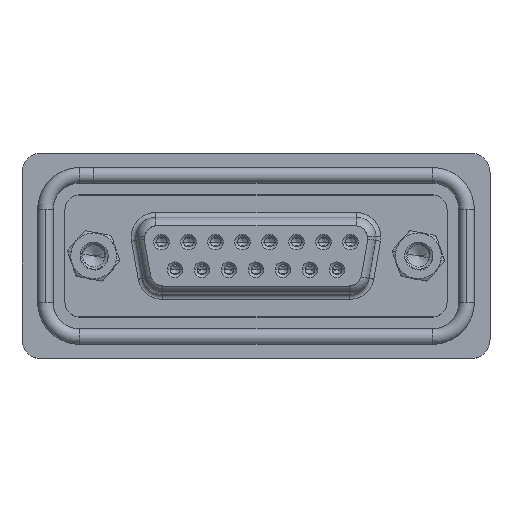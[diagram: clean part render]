
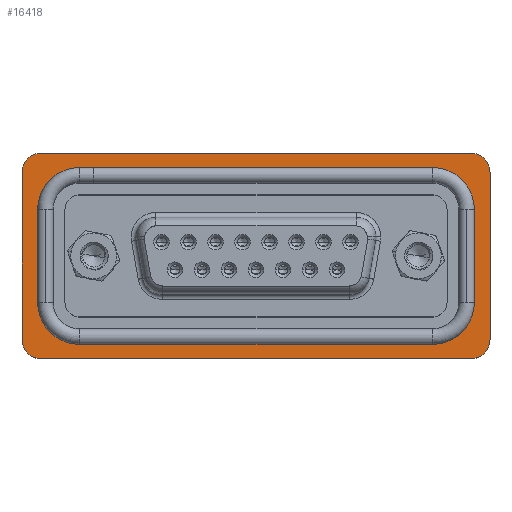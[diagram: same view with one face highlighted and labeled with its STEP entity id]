
A CAD part, top view. The second image highlights one B-rep face of the part: STEP entity #16418.
In plain terms, the highlighted planar face has unit normal (0, 0, 1).
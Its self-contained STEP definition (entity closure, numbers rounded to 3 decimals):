
#481 = VERTEX_POINT ( 'NONE', #18324 ) ;
#575 = DIRECTION ( 'NONE',  ( 1., 0., 0. ) ) ;
#1080 = CARTESIAN_POINT ( 'NONE',  ( 34.75, 9.075, 0.5 ) ) ;
#1160 = VERTEX_POINT ( 'NONE', #1566 ) ;
#1203 = CARTESIAN_POINT ( 'NONE',  ( -1.45, -9.075, 0.5 ) ) ;
#1566 = CARTESIAN_POINT ( 'NONE',  ( -5.75, 4.775, 0.5 ) ) ;
#1603 = ORIENTED_EDGE ( 'NONE', *, *, #8219, .T. ) ;
#1607 = ORIENTED_EDGE ( 'NONE', *, *, #5086, .F. ) ;
#1624 = CARTESIAN_POINT ( 'NONE',  ( -5.75, 4.775, 0.5 ) ) ;
#2034 = EDGE_CURVE ( 'NONE', #1160, #13323, #21822, .T. ) ;
#2039 = EDGE_CURVE ( 'NONE', #20120, #16101, #14316, .T. ) ;
#2099 = DIRECTION ( 'NONE',  ( 1., 0., 0. ) ) ;
#2101 = DIRECTION ( 'NONE',  ( 0., 1., 0. ) ) ;
#2139 = CIRCLE ( 'NONE', #2928, 2. ) ;
#2326 = CIRCLE ( 'NONE', #15677, 4.3 ) ;
#2415 = PLANE ( 'NONE',  #2941 ) ;
#2778 = VERTEX_POINT ( 'NONE', #7340 ) ;
#2786 = VERTEX_POINT ( 'NONE', #23828 ) ;
#2828 = DIRECTION ( 'NONE',  ( 1., 0., 0. ) ) ;
#2928 = AXIS2_PLACEMENT_3D ( 'NONE', #12668, #21630, #3425 ) ;
#2941 = AXIS2_PLACEMENT_3D ( 'NONE', #9953, #17433, #575 ) ;
#3277 = CARTESIAN_POINT ( 'NONE',  ( 40.65, 8.55, 0.5 ) ) ;
#3402 = CARTESIAN_POINT ( 'NONE',  ( 38.65, -10.55, 0.5 ) ) ;
#3425 = DIRECTION ( 'NONE',  ( -1., 0., 0. ) ) ;
#3708 = CARTESIAN_POINT ( 'NONE',  ( 40.65, -8.55, 0.5 ) ) ;
#3929 = VECTOR ( 'NONE', #2101, 1000. ) ;
#4062 = LINE ( 'NONE', #19078, #10665 ) ;
#4229 = CARTESIAN_POINT ( 'NONE',  ( 38.65, -10.55, 0.5 ) ) ;
#4257 = FACE_OUTER_BOUND ( 'NONE', #14804, .T. ) ;
#4296 = DIRECTION ( 'NONE',  ( -1., 0., 0. ) ) ;
#4420 = CARTESIAN_POINT ( 'NONE',  ( 38.65, 8.55, 0.5 ) ) ;
#4846 = DIRECTION ( 'NONE',  ( 0., 0., 1. ) ) ;
#4866 = AXIS2_PLACEMENT_3D ( 'NONE', #10271, #4846, #12354 ) ;
#4886 = ORIENTED_EDGE ( 'NONE', *, *, #23094, .T. ) ;
#5086 = EDGE_CURVE ( 'NONE', #16101, #1160, #18033, .T. ) ;
#5258 = DIRECTION ( 'NONE',  ( 1., 0., 0. ) ) ;
#5280 = AXIS2_PLACEMENT_3D ( 'NONE', #13414, #22400, #18942 ) ;
#5379 = LINE ( 'NONE', #3402, #12160 ) ;
#5762 = CARTESIAN_POINT ( 'NONE',  ( -1.45, 9.075, 0.5 ) ) ;
#5792 = EDGE_CURVE ( 'NONE', #19584, #20791, #5379, .T. ) ;
#6074 = VECTOR ( 'NONE', #11940, 1000. ) ;
#6156 = ORIENTED_EDGE ( 'NONE', *, *, #18414, .T. ) ;
#6298 = VERTEX_POINT ( 'NONE', #10416 ) ;
#6778 = DIRECTION ( 'NONE',  ( 1., 0., 0. ) ) ;
#7009 = DIRECTION ( 'NONE',  ( 1., 0., 0. ) ) ;
#7166 = EDGE_CURVE ( 'NONE', #20648, #23258, #21580, .T. ) ;
#7315 = EDGE_CURVE ( 'NONE', #13323, #2778, #2326, .T. ) ;
#7340 = CARTESIAN_POINT ( 'NONE',  ( -1.45, -9.075, 0.5 ) ) ;
#7544 = LINE ( 'NONE', #3708, #3929 ) ;
#7584 = ORIENTED_EDGE ( 'NONE', *, *, #15736, .F. ) ;
#7915 = DIRECTION ( 'NONE',  ( 0., 0., 1. ) ) ;
#8021 = CARTESIAN_POINT ( 'NONE',  ( -7.35, -8.55, 0.5 ) ) ;
#8147 = CARTESIAN_POINT ( 'NONE',  ( 39.05, -4.775, 0.5 ) ) ;
#8219 = EDGE_CURVE ( 'NONE', #22334, #20648, #7544, .T. ) ;
#8475 = VERTEX_POINT ( 'NONE', #10101 ) ;
#8505 = DIRECTION ( 'NONE',  ( 0., 0., 1. ) ) ;
#8789 = ORIENTED_EDGE ( 'NONE', *, *, #2034, .F. ) ;
#9701 = EDGE_CURVE ( 'NONE', #481, #2786, #21287, .T. ) ;
#9763 = CARTESIAN_POINT ( 'NONE',  ( -1.45, 4.775, 0.5 ) ) ;
#9953 = CARTESIAN_POINT ( 'NONE',  ( 38.65, 8.55, 0.5 ) ) ;
#9987 = CIRCLE ( 'NONE', #4866, 2. ) ;
#10093 = VERTEX_POINT ( 'NONE', #20711 ) ;
#10101 = CARTESIAN_POINT ( 'NONE',  ( -5.35, 10.55, 0.5 ) ) ;
#10135 = DIRECTION ( 'NONE',  ( 0., 0., 1. ) ) ;
#10271 = CARTESIAN_POINT ( 'NONE',  ( 38.65, -8.55, 0.5 ) ) ;
#10416 = CARTESIAN_POINT ( 'NONE',  ( -7.35, 8.55, 0.5 ) ) ;
#10665 = VECTOR ( 'NONE', #4296, 1000. ) ;
#11366 = AXIS2_PLACEMENT_3D ( 'NONE', #9763, #7915, #2828 ) ;
#11597 = DIRECTION ( 'NONE',  ( 0., -1., 0. ) ) ;
#11940 = DIRECTION ( 'NONE',  ( 0., 1., 0. ) ) ;
#11996 = EDGE_CURVE ( 'NONE', #2786, #20120, #21859, .T. ) ;
#12086 = DIRECTION ( 'NONE',  ( 1., 0., 0. ) ) ;
#12160 = VECTOR ( 'NONE', #5258, 1000. ) ;
#12203 = EDGE_CURVE ( 'NONE', #6298, #18336, #17132, .T. ) ;
#12247 = VECTOR ( 'NONE', #22064, 1000. ) ;
#12354 = DIRECTION ( 'NONE',  ( 1., 0., 0. ) ) ;
#12404 = DIRECTION ( 'NONE',  ( 0., 0., 1. ) ) ;
#12668 = CARTESIAN_POINT ( 'NONE',  ( -5.35, -8.55, 0.5 ) ) ;
#13048 = CARTESIAN_POINT ( 'NONE',  ( -5.75, -4.775, 0.5 ) ) ;
#13323 = VERTEX_POINT ( 'NONE', #13048 ) ;
#13414 = CARTESIAN_POINT ( 'NONE',  ( 34.75, -4.775, 0.5 ) ) ;
#13556 = CARTESIAN_POINT ( 'NONE',  ( -7.35, -8.55, 0.5 ) ) ;
#14253 = CARTESIAN_POINT ( 'NONE',  ( -5.35, 8.55, 0.5 ) ) ;
#14316 = LINE ( 'NONE', #23911, #12247 ) ;
#14596 = ORIENTED_EDGE ( 'NONE', *, *, #7166, .T. ) ;
#14691 = CIRCLE ( 'NONE', #21366, 2. ) ;
#14804 = EDGE_LOOP ( 'NONE', ( #14596, #6156, #4886, #20355, #20338, #22655, #21928, #1603 ) ) ;
#14974 = CARTESIAN_POINT ( 'NONE',  ( 38.65, 10.55, 0.5 ) ) ;
#15004 = ORIENTED_EDGE ( 'NONE', *, *, #2039, .F. ) ;
#15084 = EDGE_CURVE ( 'NONE', #20791, #22334, #9987, .T. ) ;
#15174 = AXIS2_PLACEMENT_3D ( 'NONE', #23417, #10135, #12086 ) ;
#15621 = DIRECTION ( 'NONE',  ( 0., 0., 1. ) ) ;
#15677 = AXIS2_PLACEMENT_3D ( 'NONE', #17831, #8505, #6778 ) ;
#15736 = EDGE_CURVE ( 'NONE', #10093, #481, #15877, .T. ) ;
#15872 = EDGE_CURVE ( 'NONE', #18336, #19584, #2139, .T. ) ;
#15877 = CIRCLE ( 'NONE', #5280, 4.3 ) ;
#15972 = VECTOR ( 'NONE', #11597, 1000. ) ;
#16101 = VERTEX_POINT ( 'NONE', #5762 ) ;
#16220 = VECTOR ( 'NONE', #23605, 1000. ) ;
#16414 = DIRECTION ( 'NONE',  ( 0., -1., 0. ) ) ;
#16418 = ADVANCED_FACE ( 'NONE', ( #17553, #4257 ), #2415, .T. ) ;
#16863 = ORIENTED_EDGE ( 'NONE', *, *, #11996, .F. ) ;
#17132 = LINE ( 'NONE', #13556, #15972 ) ;
#17433 = DIRECTION ( 'NONE',  ( 0., 0., 1. ) ) ;
#17553 = FACE_BOUND ( 'NONE', #22313, .T. ) ;
#17627 = CARTESIAN_POINT ( 'NONE',  ( -5.35, -10.55, 0.5 ) ) ;
#17831 = CARTESIAN_POINT ( 'NONE',  ( -1.45, -4.775, 0.5 ) ) ;
#17864 = ORIENTED_EDGE ( 'NONE', *, *, #9701, .F. ) ;
#17934 = LINE ( 'NONE', #1203, #16220 ) ;
#18033 = CIRCLE ( 'NONE', #11366, 4.3 ) ;
#18324 = CARTESIAN_POINT ( 'NONE',  ( 39.05, -4.775, 0.5 ) ) ;
#18336 = VERTEX_POINT ( 'NONE', #8021 ) ;
#18414 = EDGE_CURVE ( 'NONE', #23258, #8475, #4062, .T. ) ;
#18942 = DIRECTION ( 'NONE',  ( 1., 0., 0. ) ) ;
#19078 = CARTESIAN_POINT ( 'NONE',  ( 38.65, 10.55, 0.5 ) ) ;
#19584 = VERTEX_POINT ( 'NONE', #17627 ) ;
#20058 = EDGE_CURVE ( 'NONE', #2778, #10093, #17934, .T. ) ;
#20120 = VERTEX_POINT ( 'NONE', #1080 ) ;
#20338 = ORIENTED_EDGE ( 'NONE', *, *, #15872, .T. ) ;
#20355 = ORIENTED_EDGE ( 'NONE', *, *, #12203, .T. ) ;
#20648 = VERTEX_POINT ( 'NONE', #3277 ) ;
#20711 = CARTESIAN_POINT ( 'NONE',  ( 34.75, -9.075, 0.5 ) ) ;
#20791 = VERTEX_POINT ( 'NONE', #4229 ) ;
#20794 = AXIS2_PLACEMENT_3D ( 'NONE', #4420, #15621, #2099 ) ;
#21049 = ORIENTED_EDGE ( 'NONE', *, *, #7315, .F. ) ;
#21207 = ORIENTED_EDGE ( 'NONE', *, *, #20058, .F. ) ;
#21287 = LINE ( 'NONE', #8147, #6074 ) ;
#21366 = AXIS2_PLACEMENT_3D ( 'NONE', #14253, #12404, #7009 ) ;
#21580 = CIRCLE ( 'NONE', #20794, 2. ) ;
#21630 = DIRECTION ( 'NONE',  ( 0., 0., 1. ) ) ;
#21822 = LINE ( 'NONE', #1624, #23659 ) ;
#21859 = CIRCLE ( 'NONE', #15174, 4.3 ) ;
#21928 = ORIENTED_EDGE ( 'NONE', *, *, #15084, .T. ) ;
#22003 = CARTESIAN_POINT ( 'NONE',  ( 40.65, -8.55, 0.5 ) ) ;
#22064 = DIRECTION ( 'NONE',  ( -1., 0., 0. ) ) ;
#22313 = EDGE_LOOP ( 'NONE', ( #16863, #17864, #7584, #21207, #21049, #8789, #1607, #15004 ) ) ;
#22334 = VERTEX_POINT ( 'NONE', #22003 ) ;
#22400 = DIRECTION ( 'NONE',  ( 0., 0., 1. ) ) ;
#22655 = ORIENTED_EDGE ( 'NONE', *, *, #5792, .T. ) ;
#23094 = EDGE_CURVE ( 'NONE', #8475, #6298, #14691, .T. ) ;
#23258 = VERTEX_POINT ( 'NONE', #14974 ) ;
#23417 = CARTESIAN_POINT ( 'NONE',  ( 34.75, 4.775, 0.5 ) ) ;
#23605 = DIRECTION ( 'NONE',  ( 1., 0., 0. ) ) ;
#23659 = VECTOR ( 'NONE', #16414, 1000. ) ;
#23828 = CARTESIAN_POINT ( 'NONE',  ( 39.05, 4.775, 0.5 ) ) ;
#23911 = CARTESIAN_POINT ( 'NONE',  ( 34.75, 9.075, 0.5 ) ) ;
